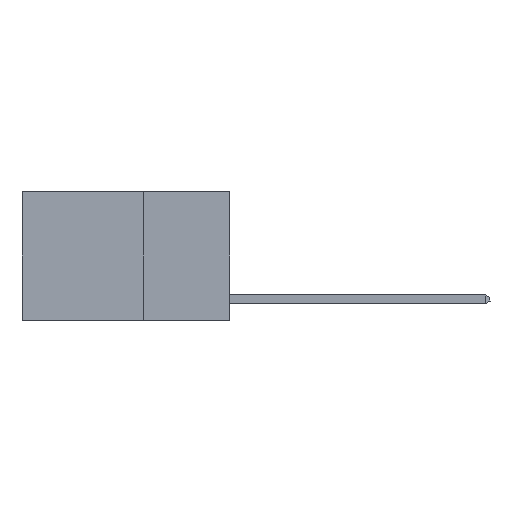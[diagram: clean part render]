
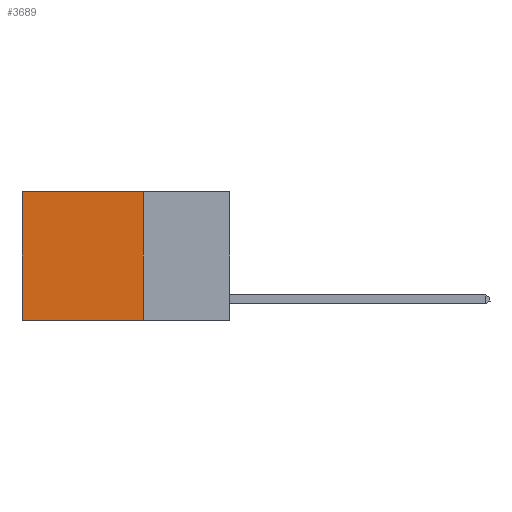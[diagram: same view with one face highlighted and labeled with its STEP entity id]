
A CAD part, left-side view. The second image highlights one B-rep face of the part: STEP entity #3689.
In plain terms, the highlighted planar face has unit normal (-1, 0, 0).
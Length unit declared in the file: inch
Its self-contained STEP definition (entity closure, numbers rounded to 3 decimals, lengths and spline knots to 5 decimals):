
#351 = DIRECTION ( 'NONE',  ( 0., 0., -1. ) ) ;
#1619 = VECTOR ( 'NONE', #351, 39.37008 ) ;
#1646 = CARTESIAN_POINT ( 'NONE',  ( 0.2625, 0.25, 0. ) ) ;
#3030 = LINE ( 'NONE', #10163, #11120 ) ;
#3131 = ORIENTED_EDGE ( 'NONE', *, *, #12363, .F. ) ;
#3406 = AXIS2_PLACEMENT_3D ( 'NONE', #3525, #3624, #3664 ) ;
#3525 = CARTESIAN_POINT ( 'NONE',  ( 0.2625, 0.25, 0. ) ) ;
#3624 = DIRECTION ( 'NONE',  ( 1., 0., 0. ) ) ;
#3664 = DIRECTION ( 'NONE',  ( 0., 0., -1. ) ) ;
#3678 = CARTESIAN_POINT ( 'NONE',  ( 0.2625, 0.25, 0. ) ) ;
#3689 = ADVANCED_FACE ( 'NONE', ( #12582 ), #4499, .F. ) ;
#3748 = EDGE_CURVE ( 'NONE', #7094, #6652, #3832, .T. ) ;
#3832 = LINE ( 'NONE', #1646, #4335 ) ;
#3906 = ORIENTED_EDGE ( 'NONE', *, *, #3748, .T. ) ;
#3918 = LINE ( 'NONE', #6667, #1619 ) ;
#4335 = VECTOR ( 'NONE', #9139, 39.37008 ) ;
#4499 = PLANE ( 'NONE',  #3406 ) ;
#4991 = CARTESIAN_POINT ( 'NONE',  ( 0.2625, 0.25, -0.37 ) ) ;
#5176 = CARTESIAN_POINT ( 'NONE',  ( 0.2625, 0.6, -0.37 ) ) ;
#6000 = DIRECTION ( 'NONE',  ( 0., 1., 0. ) ) ;
#6350 = EDGE_LOOP ( 'NONE', ( #10688, #13239, #3131, #3906 ) ) ;
#6652 = VERTEX_POINT ( 'NONE', #8625 ) ;
#6667 = CARTESIAN_POINT ( 'NONE',  ( 0.2625, 0.6, 0. ) ) ;
#7094 = VERTEX_POINT ( 'NONE', #9207 ) ;
#7906 = EDGE_CURVE ( 'NONE', #12538, #12534, #3030, .T. ) ;
#8625 = CARTESIAN_POINT ( 'NONE',  ( 0.2625, 0.6, 0. ) ) ;
#8721 = VECTOR ( 'NONE', #9021, 39.37008 ) ;
#9021 = DIRECTION ( 'NONE',  ( 0., 0., -1. ) ) ;
#9139 = DIRECTION ( 'NONE',  ( 0., 1., 0. ) ) ;
#9207 = CARTESIAN_POINT ( 'NONE',  ( 0.2625, 0.25, 0. ) ) ;
#10163 = CARTESIAN_POINT ( 'NONE',  ( 0.2625, 0.25, -0.37 ) ) ;
#10524 = LINE ( 'NONE', #3678, #8721 ) ;
#10688 = ORIENTED_EDGE ( 'NONE', *, *, #12823, .T. ) ;
#11120 = VECTOR ( 'NONE', #6000, 39.37008 ) ;
#12363 = EDGE_CURVE ( 'NONE', #7094, #12538, #10524, .T. ) ;
#12534 = VERTEX_POINT ( 'NONE', #5176 ) ;
#12538 = VERTEX_POINT ( 'NONE', #4991 ) ;
#12582 = FACE_OUTER_BOUND ( 'NONE', #6350, .T. ) ;
#12823 = EDGE_CURVE ( 'NONE', #6652, #12534, #3918, .T. ) ;
#13239 = ORIENTED_EDGE ( 'NONE', *, *, #7906, .F. ) ;
